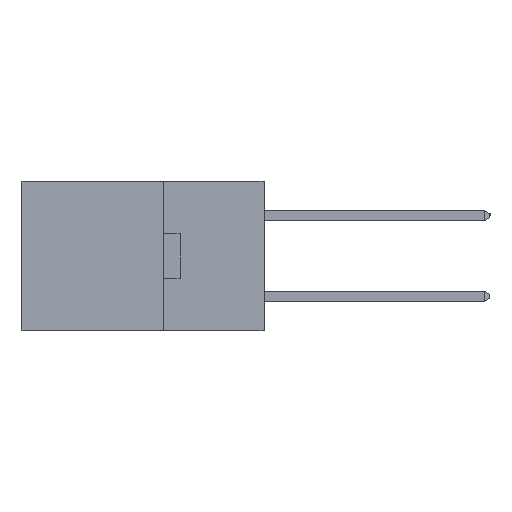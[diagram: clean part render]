
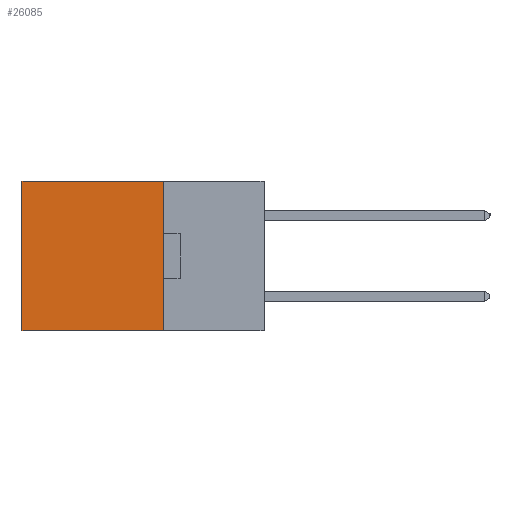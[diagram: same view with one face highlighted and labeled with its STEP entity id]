
A CAD part, left-side view. The second image highlights one B-rep face of the part: STEP entity #26085.
In plain terms, the highlighted planar face has unit normal (-1, 0, 0).
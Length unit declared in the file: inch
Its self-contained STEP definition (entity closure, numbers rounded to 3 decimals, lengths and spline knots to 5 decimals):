
#1181 = CARTESIAN_POINT ( 'NONE',  ( 0.2615, 0.25, 0. ) ) ;
#1401 = DIRECTION ( 'NONE',  ( 0., 0., -1. ) ) ;
#2309 = ORIENTED_EDGE ( 'NONE', *, *, #28361, .F. ) ;
#2888 = VERTEX_POINT ( 'NONE', #26742 ) ;
#3365 = LINE ( 'NONE', #10063, #4375 ) ;
#4102 = EDGE_CURVE ( 'NONE', #21560, #2888, #18338, .T. ) ;
#4375 = VECTOR ( 'NONE', #19131, 39.37008 ) ;
#5604 = DIRECTION ( 'NONE',  ( 1., 0., 0. ) ) ;
#8087 = PLANE ( 'NONE',  #11838 ) ;
#8324 = VERTEX_POINT ( 'NONE', #18933 ) ;
#9708 = EDGE_CURVE ( 'NONE', #8324, #11159, #24954, .T. ) ;
#10063 = CARTESIAN_POINT ( 'NONE',  ( 0.2615, 0.25, -0.37 ) ) ;
#10066 = DIRECTION ( 'NONE',  ( 0., 0., -1. ) ) ;
#10095 = VECTOR ( 'NONE', #13652, 39.37008 ) ;
#11159 = VERTEX_POINT ( 'NONE', #18556 ) ;
#11838 = AXIS2_PLACEMENT_3D ( 'NONE', #18772, #5604, #1401 ) ;
#12338 = FACE_OUTER_BOUND ( 'NONE', #18341, .T. ) ;
#12553 = CARTESIAN_POINT ( 'NONE',  ( 0.2615, 0.6, -0.37 ) ) ;
#13652 = DIRECTION ( 'NONE',  ( 0., 1., 0. ) ) ;
#13999 = CARTESIAN_POINT ( 'NONE',  ( 0.2615, 0.25, -0.37 ) ) ;
#14009 = DIRECTION ( 'NONE',  ( 0., 1., 0. ) ) ;
#15020 = ORIENTED_EDGE ( 'NONE', *, *, #4102, .F. ) ;
#18338 = LINE ( 'NONE', #27346, #10095 ) ;
#18341 = EDGE_LOOP ( 'NONE', ( #21667, #15020, #2309, #25583 ) ) ;
#18556 = CARTESIAN_POINT ( 'NONE',  ( 0.2615, 0.6, 0. ) ) ;
#18772 = CARTESIAN_POINT ( 'NONE',  ( 0.2615, 0.25, -0.37 ) ) ;
#18933 = CARTESIAN_POINT ( 'NONE',  ( 0.2615, 0.25, 0. ) ) ;
#19131 = DIRECTION ( 'NONE',  ( 0., 0., -1. ) ) ;
#21195 = EDGE_CURVE ( 'NONE', #11159, #2888, #28151, .T. ) ;
#21560 = VERTEX_POINT ( 'NONE', #13999 ) ;
#21667 = ORIENTED_EDGE ( 'NONE', *, *, #21195, .T. ) ;
#24190 = VECTOR ( 'NONE', #10066, 39.37008 ) ;
#24799 = VECTOR ( 'NONE', #14009, 39.37008 ) ;
#24954 = LINE ( 'NONE', #1181, #24799 ) ;
#25583 = ORIENTED_EDGE ( 'NONE', *, *, #9708, .T. ) ;
#26085 = ADVANCED_FACE ( 'NONE', ( #12338 ), #8087, .F. ) ;
#26742 = CARTESIAN_POINT ( 'NONE',  ( 0.2615, 0.6, -0.37 ) ) ;
#27346 = CARTESIAN_POINT ( 'NONE',  ( 0.2615, 0.25, -0.37 ) ) ;
#28151 = LINE ( 'NONE', #12553, #24190 ) ;
#28361 = EDGE_CURVE ( 'NONE', #8324, #21560, #3365, .T. ) ;
